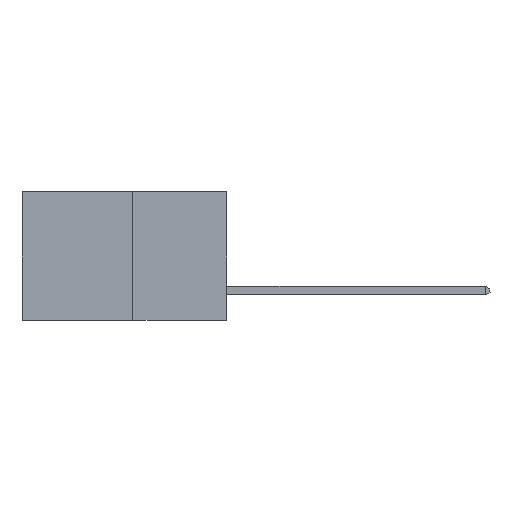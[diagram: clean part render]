
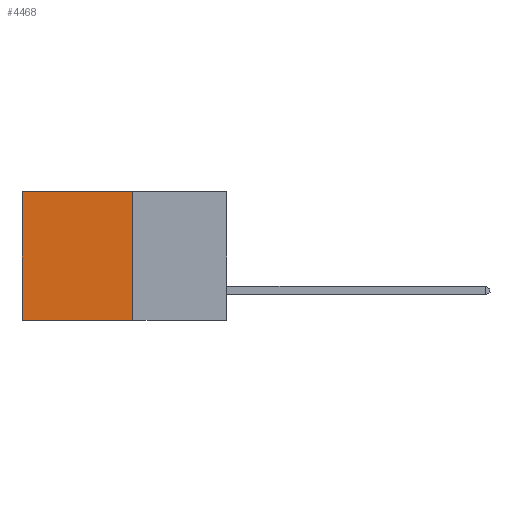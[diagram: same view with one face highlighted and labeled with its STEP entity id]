
A CAD part, left-side view. The second image highlights one B-rep face of the part: STEP entity #4468.
In plain terms, the highlighted planar face has unit normal (-1, 0, 0).
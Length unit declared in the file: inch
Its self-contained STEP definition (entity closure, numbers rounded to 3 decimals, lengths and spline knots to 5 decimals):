
#939 = DIRECTION ( 'NONE',  ( 0., 1., 0. ) ) ;
#1033 = EDGE_CURVE ( 'NONE', #5574, #6006, #8516, .T. ) ;
#1316 = DIRECTION ( 'NONE',  ( 0., 0., -1. ) ) ;
#1856 = VECTOR ( 'NONE', #9560, 39.37008 ) ;
#2066 = ORIENTED_EDGE ( 'NONE', *, *, #7429, .T. ) ;
#2758 = VERTEX_POINT ( 'NONE', #6954 ) ;
#2828 = DIRECTION ( 'NONE',  ( 0., 0., -1. ) ) ;
#2902 = VERTEX_POINT ( 'NONE', #5314 ) ;
#3228 = ORIENTED_EDGE ( 'NONE', *, *, #1033, .T. ) ;
#4176 = VECTOR ( 'NONE', #2828, 39.37008 ) ;
#4468 = ADVANCED_FACE ( 'NONE', ( #9935 ), #10875, .F. ) ;
#4571 = EDGE_CURVE ( 'NONE', #2902, #2758, #8932, .T. ) ;
#4783 = AXIS2_PLACEMENT_3D ( 'NONE', #11145, #10839, #10801 ) ;
#5314 = CARTESIAN_POINT ( 'NONE',  ( 0.277, 0.27, -0.37 ) ) ;
#5574 = VERTEX_POINT ( 'NONE', #9880 ) ;
#5695 = CARTESIAN_POINT ( 'NONE',  ( 0.277, 0.59, 0. ) ) ;
#6006 = VERTEX_POINT ( 'NONE', #5695 ) ;
#6282 = VECTOR ( 'NONE', #939, 39.37008 ) ;
#6586 = LINE ( 'NONE', #7358, #4176 ) ;
#6954 = CARTESIAN_POINT ( 'NONE',  ( 0.277, 0.59, -0.37 ) ) ;
#7035 = EDGE_LOOP ( 'NONE', ( #2066, #9099, #9361, #3228 ) ) ;
#7358 = CARTESIAN_POINT ( 'NONE',  ( 0.277, 0.59, -0.37 ) ) ;
#7429 = EDGE_CURVE ( 'NONE', #6006, #2758, #6586, .T. ) ;
#7710 = CARTESIAN_POINT ( 'NONE',  ( 0.277, 0.27, -0.37 ) ) ;
#7778 = CARTESIAN_POINT ( 'NONE',  ( 0.277, 0.27, 0. ) ) ;
#8516 = LINE ( 'NONE', #7778, #6282 ) ;
#8932 = LINE ( 'NONE', #9358, #1856 ) ;
#8967 = VECTOR ( 'NONE', #1316, 39.37008 ) ;
#9099 = ORIENTED_EDGE ( 'NONE', *, *, #4571, .F. ) ;
#9358 = CARTESIAN_POINT ( 'NONE',  ( 0.277, 0.27, -0.37 ) ) ;
#9361 = ORIENTED_EDGE ( 'NONE', *, *, #10751, .F. ) ;
#9560 = DIRECTION ( 'NONE',  ( 0., 1., 0. ) ) ;
#9880 = CARTESIAN_POINT ( 'NONE',  ( 0.277, 0.27, 0. ) ) ;
#9935 = FACE_OUTER_BOUND ( 'NONE', #7035, .T. ) ;
#10751 = EDGE_CURVE ( 'NONE', #5574, #2902, #11373, .T. ) ;
#10801 = DIRECTION ( 'NONE',  ( 0., 0., -1. ) ) ;
#10839 = DIRECTION ( 'NONE',  ( 1., 0., 0. ) ) ;
#10875 = PLANE ( 'NONE',  #4783 ) ;
#11145 = CARTESIAN_POINT ( 'NONE',  ( 0.277, 0.27, -0.37 ) ) ;
#11373 = LINE ( 'NONE', #7710, #8967 ) ;
